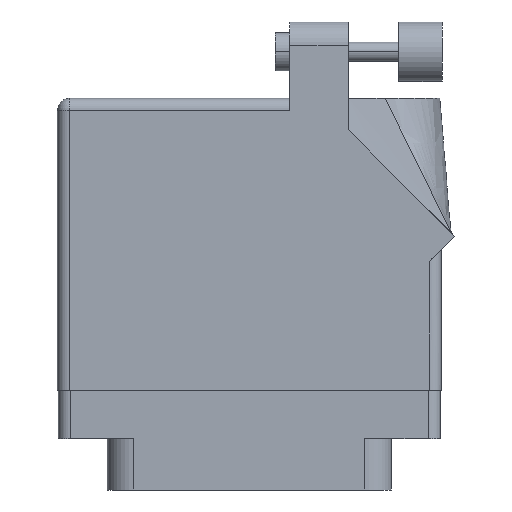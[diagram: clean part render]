
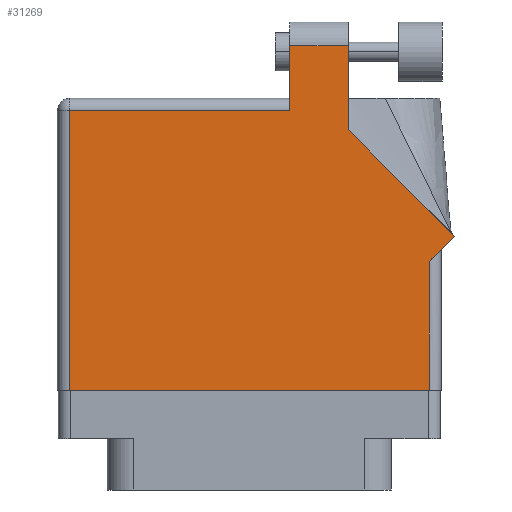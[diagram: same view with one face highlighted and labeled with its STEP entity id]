
A CAD part, front view. The second image highlights one B-rep face of the part: STEP entity #31269.
In plain terms, the highlighted face is planar.
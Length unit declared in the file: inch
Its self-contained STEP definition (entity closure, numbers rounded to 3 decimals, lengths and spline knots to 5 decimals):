
#52 = LINE ( 'NONE', #36067, #13137 ) ;
#383 = VECTOR ( 'NONE', #9464, 39.37008 ) ;
#1128 = CARTESIAN_POINT ( 'NONE',  ( -0.943, 1.368, 0.455 ) ) ;
#1649 = EDGE_CURVE ( 'NONE', #1678, #9204, #5657, .T. ) ;
#1678 = VERTEX_POINT ( 'NONE', #3394 ) ;
#1702 = CARTESIAN_POINT ( 'NONE',  ( -1.005, -0.1, 0.455 ) ) ;
#1824 = DIRECTION ( 'NONE',  ( 1., 0., 0. ) ) ;
#2114 = EDGE_CURVE ( 'NONE', #6805, #29104, #15207, .T. ) ;
#2196 = ORIENTED_EDGE ( 'NONE', *, *, #24745, .T. ) ;
#2666 = CARTESIAN_POINT ( 'NONE',  ( -0.943, -0.1, 0.455 ) ) ;
#3394 = CARTESIAN_POINT ( 'NONE',  ( 0.212, 1.705, 0.455 ) ) ;
#3512 = CARTESIAN_POINT ( 'NONE',  ( -1.005, 1.368, 0.455 ) ) ;
#4053 = LINE ( 'NONE', #1702, #13216 ) ;
#4072 = DIRECTION ( 'NONE',  ( 0., 1., 0. ) ) ;
#4078 = ORIENTED_EDGE ( 'NONE', *, *, #23949, .T. ) ;
#4675 = ORIENTED_EDGE ( 'NONE', *, *, #1649, .T. ) ;
#4981 = VECTOR ( 'NONE', #7187, 39.37008 ) ;
#5657 = LINE ( 'NONE', #20429, #383 ) ;
#6060 = DIRECTION ( 'NONE',  ( 0., 1., 0. ) ) ;
#6599 = DIRECTION ( 'NONE',  ( 0., 0., -1. ) ) ;
#6711 = PLANE ( 'NONE',  #16652 ) ;
#6805 = VERTEX_POINT ( 'NONE', #6817 ) ;
#6817 = CARTESIAN_POINT ( 'NONE',  ( 0.943, -0.1, 0.455 ) ) ;
#6826 = VERTEX_POINT ( 'NONE', #23965 ) ;
#7187 = DIRECTION ( 'NONE',  ( 0.707, 0.707, 0. ) ) ;
#7309 = VECTOR ( 'NONE', #6060, 39.37008 ) ;
#7387 = CARTESIAN_POINT ( 'NONE',  ( 0.519, 1.705, 0.455 ) ) ;
#7985 = ORIENTED_EDGE ( 'NONE', *, *, #19820, .T. ) ;
#8981 = ORIENTED_EDGE ( 'NONE', *, *, #2114, .T. ) ;
#9204 = VERTEX_POINT ( 'NONE', #34389 ) ;
#9464 = DIRECTION ( 'NONE',  ( 0., -1., 0. ) ) ;
#10926 = DIRECTION ( 'NONE',  ( -1., 0., 0. ) ) ;
#11175 = EDGE_CURVE ( 'NONE', #9204, #17028, #30086, .T. ) ;
#11202 = DIRECTION ( 'NONE',  ( 0., -1., 0. ) ) ;
#12413 = LINE ( 'NONE', #15680, #28547 ) ;
#13047 = DIRECTION ( 'NONE',  ( -1., 0., 0. ) ) ;
#13137 = VECTOR ( 'NONE', #10926, 39.37008 ) ;
#13216 = VECTOR ( 'NONE', #1824, 39.37008 ) ;
#13633 = EDGE_CURVE ( 'NONE', #29995, #1678, #52, .T. ) ;
#15207 = LINE ( 'NONE', #25551, #7309 ) ;
#15430 = EDGE_CURVE ( 'NONE', #17028, #22391, #23840, .T. ) ;
#15680 = CARTESIAN_POINT ( 'NONE',  ( 0.519, 1.26442, 0.455 ) ) ;
#15830 = VECTOR ( 'NONE', #35223, 39.37008 ) ;
#15850 = CARTESIAN_POINT ( 'NONE',  ( 1.07571, 0.70771, 0.455 ) ) ;
#16328 = LINE ( 'NONE', #32177, #4981 ) ;
#16652 = AXIS2_PLACEMENT_3D ( 'NONE', #20689, #6599, #13047 ) ;
#17028 = VERTEX_POINT ( 'NONE', #1128 ) ;
#17096 = ORIENTED_EDGE ( 'NONE', *, *, #24627, .T. ) ;
#17373 = FACE_OUTER_BOUND ( 'NONE', #32222, .T. ) ;
#17423 = CARTESIAN_POINT ( 'NONE',  ( 0.519, 1.26442, 0.455 ) ) ;
#18989 = ORIENTED_EDGE ( 'NONE', *, *, #15430, .T. ) ;
#19820 = EDGE_CURVE ( 'NONE', #6826, #31639, #31922, .T. ) ;
#20429 = CARTESIAN_POINT ( 'NONE',  ( 0.212, 1.43, 0.455 ) ) ;
#20689 = CARTESIAN_POINT ( 'NONE',  ( -1.005, 1.43, 0.455 ) ) ;
#22391 = VERTEX_POINT ( 'NONE', #35517 ) ;
#23840 = LINE ( 'NONE', #2666, #30435 ) ;
#23949 = EDGE_CURVE ( 'NONE', #31639, #29995, #12413, .T. ) ;
#23965 = CARTESIAN_POINT ( 'NONE',  ( 1.07571, 0.70771, 0.455 ) ) ;
#24627 = EDGE_CURVE ( 'NONE', #29104, #6826, #16328, .T. ) ;
#24745 = EDGE_CURVE ( 'NONE', #22391, #6805, #4053, .T. ) ;
#24826 = VECTOR ( 'NONE', #31675, 39.37008 ) ;
#25551 = CARTESIAN_POINT ( 'NONE',  ( 0.943, 0.637, 0.455 ) ) ;
#28547 = VECTOR ( 'NONE', #4072, 39.37008 ) ;
#29104 = VERTEX_POINT ( 'NONE', #30948 ) ;
#29995 = VERTEX_POINT ( 'NONE', #7387 ) ;
#30086 = LINE ( 'NONE', #3512, #24826 ) ;
#30435 = VECTOR ( 'NONE', #11202, 39.37008 ) ;
#30948 = CARTESIAN_POINT ( 'NONE',  ( 0.943, 0.575, 0.455 ) ) ;
#31269 = ADVANCED_FACE ( 'NONE', ( #17373 ), #6711, .F. ) ;
#31284 = ORIENTED_EDGE ( 'NONE', *, *, #11175, .T. ) ;
#31639 = VERTEX_POINT ( 'NONE', #17423 ) ;
#31675 = DIRECTION ( 'NONE',  ( -1., 0., 0. ) ) ;
#31922 = LINE ( 'NONE', #15850, #15830 ) ;
#32177 = CARTESIAN_POINT ( 'NONE',  ( 1.005, 0.637, 0.455 ) ) ;
#32222 = EDGE_LOOP ( 'NONE', ( #4078, #32518, #4675, #31284, #18989, #2196, #8981, #17096, #7985 ) ) ;
#32518 = ORIENTED_EDGE ( 'NONE', *, *, #13633, .T. ) ;
#34389 = CARTESIAN_POINT ( 'NONE',  ( 0.212, 1.368, 0.455 ) ) ;
#35223 = DIRECTION ( 'NONE',  ( -0.707, 0.707, 0. ) ) ;
#35517 = CARTESIAN_POINT ( 'NONE',  ( -0.943, -0.1, 0.455 ) ) ;
#36067 = CARTESIAN_POINT ( 'NONE',  ( 0.212, 1.705, 0.455 ) ) ;
